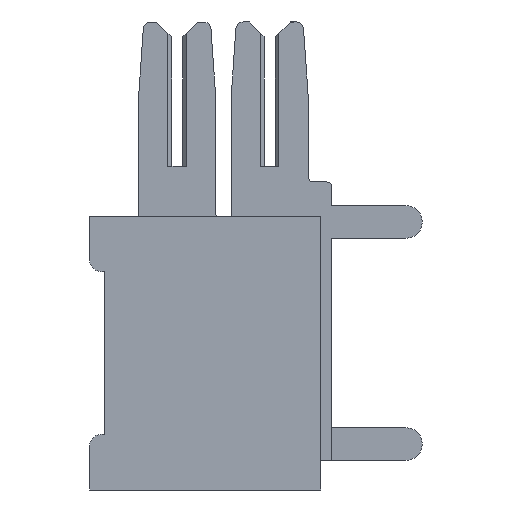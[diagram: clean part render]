
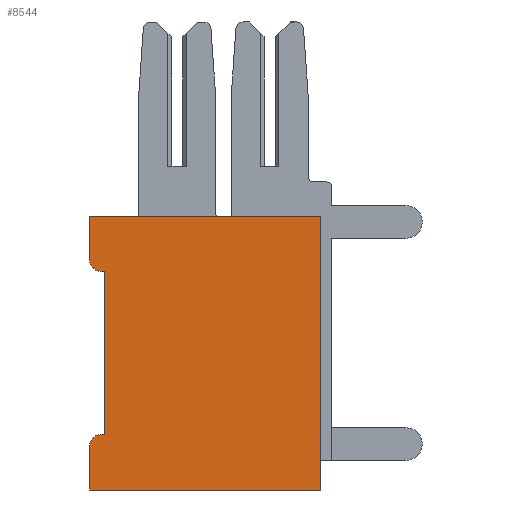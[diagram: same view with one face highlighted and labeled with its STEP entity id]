
A CAD part, left-side view. The second image highlights one B-rep face of the part: STEP entity #8544.
In plain terms, the highlighted planar face has unit normal (-1, 0, 0).
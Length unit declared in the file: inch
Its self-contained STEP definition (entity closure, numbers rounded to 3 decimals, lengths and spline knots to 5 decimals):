
#3 = CARTESIAN_POINT ( 'NONE',  ( 0., 0., -0.37 ) ) ;
#251 = DIRECTION ( 'NONE',  ( 0., 0., 1. ) ) ;
#531 = CARTESIAN_POINT ( 'NONE',  ( 0., 0.312, -0.075 ) ) ;
#579 = CARTESIAN_POINT ( 'NONE',  ( 0., 0.297, -0.06 ) ) ;
#582 = LINE ( 'NONE', #3, #8198 ) ;
#623 = ORIENTED_EDGE ( 'NONE', *, *, #5670, .T. ) ;
#819 = ORIENTED_EDGE ( 'NONE', *, *, #1878, .F. ) ;
#969 = CARTESIAN_POINT ( 'NONE',  ( 0., 0.312, -0.37 ) ) ;
#1107 = DIRECTION ( 'NONE',  ( 0., 0., 1. ) ) ;
#1172 = LINE ( 'NONE', #531, #4720 ) ;
#1645 = CARTESIAN_POINT ( 'NONE',  ( 0., 0.312, -0.31 ) ) ;
#1696 = ORIENTED_EDGE ( 'NONE', *, *, #6775, .T. ) ;
#1765 = AXIS2_PLACEMENT_3D ( 'NONE', #2762, #7920, #251 ) ;
#1878 = EDGE_CURVE ( 'NONE', #2966, #2415, #1172, .T. ) ;
#1918 = CIRCLE ( 'NONE', #6187, 0.015 ) ;
#2028 = CARTESIAN_POINT ( 'NONE',  ( 0., 0.297, -0.295 ) ) ;
#2154 = ORIENTED_EDGE ( 'NONE', *, *, #7029, .F. ) ;
#2353 = EDGE_CURVE ( 'NONE', #5873, #8442, #2874, .T. ) ;
#2415 = VERTEX_POINT ( 'NONE', #2915 ) ;
#2421 = LINE ( 'NONE', #3037, #6890 ) ;
#2563 = EDGE_CURVE ( 'NONE', #4627, #7259, #10704, .T. ) ;
#2677 = CARTESIAN_POINT ( 'NONE',  ( 0., 0., -0.37 ) ) ;
#2729 = VECTOR ( 'NONE', #10217, 39.37008 ) ;
#2762 = CARTESIAN_POINT ( 'NONE',  ( 0., 0., -0.37 ) ) ;
#2839 = VERTEX_POINT ( 'NONE', #2028 ) ;
#2874 = LINE ( 'NONE', #969, #8770 ) ;
#2915 = CARTESIAN_POINT ( 'NONE',  ( 0., 0.297, -0.075 ) ) ;
#2966 = VERTEX_POINT ( 'NONE', #5610 ) ;
#3037 = CARTESIAN_POINT ( 'NONE',  ( 0., 0.312, -0.295 ) ) ;
#3078 = DIRECTION ( 'NONE',  ( 0., 1., 0. ) ) ;
#3122 = DIRECTION ( 'NONE',  ( -1., 0., 0. ) ) ;
#3218 = LINE ( 'NONE', #3828, #10528 ) ;
#3384 = ORIENTED_EDGE ( 'NONE', *, *, #7760, .F. ) ;
#3403 = FACE_OUTER_BOUND ( 'NONE', #5827, .T. ) ;
#3418 = CARTESIAN_POINT ( 'NONE',  ( 0., 0., -0.37 ) ) ;
#3570 = CARTESIAN_POINT ( 'NONE',  ( 0., 0.292, -0.295 ) ) ;
#3698 = DIRECTION ( 'NONE',  ( 0., 0., 1. ) ) ;
#3828 = CARTESIAN_POINT ( 'NONE',  ( 0., 0., 0. ) ) ;
#4009 = CARTESIAN_POINT ( 'NONE',  ( 0., 0., 0. ) ) ;
#4162 = CIRCLE ( 'NONE', #4229, 0.015 ) ;
#4229 = AXIS2_PLACEMENT_3D ( 'NONE', #579, #3122, #9861 ) ;
#4627 = VERTEX_POINT ( 'NONE', #3418 ) ;
#4705 = VECTOR ( 'NONE', #5219, 39.37008 ) ;
#4720 = VECTOR ( 'NONE', #3078, 39.37008 ) ;
#4732 = CARTESIAN_POINT ( 'NONE',  ( 0., 0.312, -0.37 ) ) ;
#4882 = ORIENTED_EDGE ( 'NONE', *, *, #2563, .T. ) ;
#5219 = DIRECTION ( 'NONE',  ( 0., 0., 1. ) ) ;
#5302 = PLANE ( 'NONE',  #1765 ) ;
#5363 = DIRECTION ( 'NONE',  ( -1., 0., 0. ) ) ;
#5401 = CARTESIAN_POINT ( 'NONE',  ( 0., 0.297, -0.31 ) ) ;
#5610 = CARTESIAN_POINT ( 'NONE',  ( 0., 0.292, -0.075 ) ) ;
#5670 = EDGE_CURVE ( 'NONE', #2839, #8311, #1918, .T. ) ;
#5827 = EDGE_LOOP ( 'NONE', ( #10780, #6017, #819, #6439, #7046, #623, #3384, #1696, #4882, #2154 ) ) ;
#5873 = VERTEX_POINT ( 'NONE', #9020 ) ;
#5970 = CARTESIAN_POINT ( 'NONE',  ( 0., 0.312, 0. ) ) ;
#6017 = ORIENTED_EDGE ( 'NONE', *, *, #8911, .T. ) ;
#6187 = AXIS2_PLACEMENT_3D ( 'NONE', #5401, #5363, #3698 ) ;
#6431 = EDGE_CURVE ( 'NONE', #2839, #10740, #2421, .T. ) ;
#6439 = ORIENTED_EDGE ( 'NONE', *, *, #8342, .F. ) ;
#6543 = CARTESIAN_POINT ( 'NONE',  ( 0., 0.292, -0.295 ) ) ;
#6775 = EDGE_CURVE ( 'NONE', #8879, #4627, #582, .T. ) ;
#6828 = VECTOR ( 'NONE', #8844, 39.37008 ) ;
#6890 = VECTOR ( 'NONE', #8791, 39.37008 ) ;
#7029 = EDGE_CURVE ( 'NONE', #8442, #7259, #3218, .T. ) ;
#7046 = ORIENTED_EDGE ( 'NONE', *, *, #6431, .F. ) ;
#7259 = VERTEX_POINT ( 'NONE', #4009 ) ;
#7337 = CARTESIAN_POINT ( 'NONE',  ( 0., 0.312, -0.37 ) ) ;
#7540 = DIRECTION ( 'NONE',  ( 0., -1., 0. ) ) ;
#7760 = EDGE_CURVE ( 'NONE', #8879, #8311, #8797, .T. ) ;
#7920 = DIRECTION ( 'NONE',  ( -1., 0., 0. ) ) ;
#8198 = VECTOR ( 'NONE', #7540, 39.37008 ) ;
#8311 = VERTEX_POINT ( 'NONE', #1645 ) ;
#8342 = EDGE_CURVE ( 'NONE', #10740, #2966, #8641, .T. ) ;
#8442 = VERTEX_POINT ( 'NONE', #5970 ) ;
#8544 = ADVANCED_FACE ( 'NONE', ( #3403 ), #5302, .T. ) ;
#8641 = LINE ( 'NONE', #3570, #4705 ) ;
#8770 = VECTOR ( 'NONE', #1107, 39.37008 ) ;
#8791 = DIRECTION ( 'NONE',  ( 0., -1., 0. ) ) ;
#8797 = LINE ( 'NONE', #4732, #6828 ) ;
#8844 = DIRECTION ( 'NONE',  ( 0., 0., 1. ) ) ;
#8879 = VERTEX_POINT ( 'NONE', #7337 ) ;
#8911 = EDGE_CURVE ( 'NONE', #5873, #2415, #4162, .T. ) ;
#9020 = CARTESIAN_POINT ( 'NONE',  ( 0., 0.312, -0.06 ) ) ;
#9698 = DIRECTION ( 'NONE',  ( 0., -1., 0. ) ) ;
#9861 = DIRECTION ( 'NONE',  ( 0., 0., 1. ) ) ;
#10217 = DIRECTION ( 'NONE',  ( 0., 0., 1. ) ) ;
#10528 = VECTOR ( 'NONE', #9698, 39.37008 ) ;
#10704 = LINE ( 'NONE', #2677, #2729 ) ;
#10740 = VERTEX_POINT ( 'NONE', #6543 ) ;
#10780 = ORIENTED_EDGE ( 'NONE', *, *, #2353, .F. ) ;
